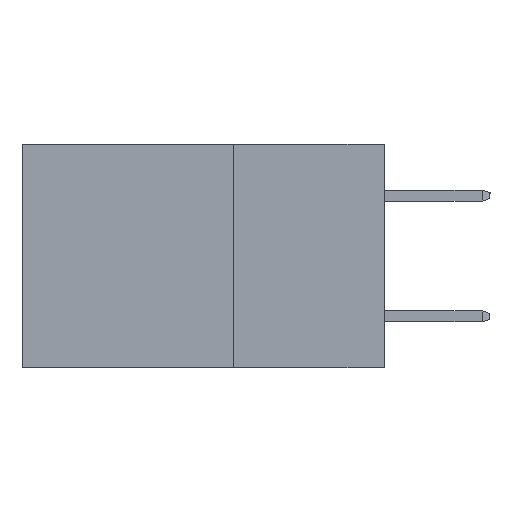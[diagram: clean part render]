
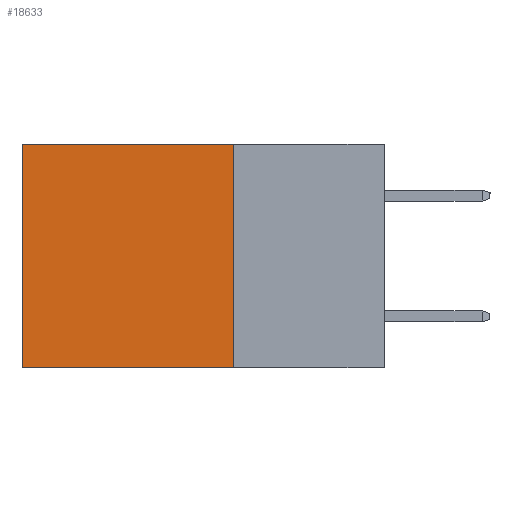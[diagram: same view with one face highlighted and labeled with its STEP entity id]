
A CAD part, left-side view. The second image highlights one B-rep face of the part: STEP entity #18633.
In plain terms, the highlighted planar face has unit normal (-1, 0, 0).
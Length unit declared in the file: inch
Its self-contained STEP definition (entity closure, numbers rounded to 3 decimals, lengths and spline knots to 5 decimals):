
#569 = EDGE_CURVE ( 'NONE', #25233, #17276, #4604, .T. ) ;
#2341 = CARTESIAN_POINT ( 'NONE',  ( 0.2615, 0.6, 0. ) ) ;
#3344 = LINE ( 'NONE', #7152, #25941 ) ;
#3527 = CARTESIAN_POINT ( 'NONE',  ( 0.2615, 0.25, -0.37 ) ) ;
#4604 = LINE ( 'NONE', #23424, #6403 ) ;
#4832 = VECTOR ( 'NONE', #15853, 39.37008 ) ;
#4960 = CARTESIAN_POINT ( 'NONE',  ( 0.2615, 0.6, -0.37 ) ) ;
#5496 = EDGE_CURVE ( 'NONE', #25233, #19333, #7345, .T. ) ;
#5846 = DIRECTION ( 'NONE',  ( 0., 0., -1. ) ) ;
#6215 = EDGE_LOOP ( 'NONE', ( #10912, #23423, #11463, #14062 ) ) ;
#6403 = VECTOR ( 'NONE', #12867, 39.37008 ) ;
#7152 = CARTESIAN_POINT ( 'NONE',  ( 0.2615, 0.25, -0.37 ) ) ;
#7345 = LINE ( 'NONE', #3527, #4832 ) ;
#7699 = DIRECTION ( 'NONE',  ( 0., 1., 0. ) ) ;
#9401 = LINE ( 'NONE', #24568, #17720 ) ;
#10912 = ORIENTED_EDGE ( 'NONE', *, *, #14545, .T. ) ;
#11463 = ORIENTED_EDGE ( 'NONE', *, *, #5496, .F. ) ;
#12867 = DIRECTION ( 'NONE',  ( 0., 1., 0. ) ) ;
#14057 = EDGE_CURVE ( 'NONE', #19333, #22505, #3344, .T. ) ;
#14062 = ORIENTED_EDGE ( 'NONE', *, *, #569, .T. ) ;
#14545 = EDGE_CURVE ( 'NONE', #17276, #22505, #9401, .T. ) ;
#15853 = DIRECTION ( 'NONE',  ( 0., 0., -1. ) ) ;
#17276 = VERTEX_POINT ( 'NONE', #2341 ) ;
#17720 = VECTOR ( 'NONE', #20624, 39.37008 ) ;
#18430 = PLANE ( 'NONE',  #20411 ) ;
#18633 = ADVANCED_FACE ( 'NONE', ( #22371 ), #18430, .F. ) ;
#19333 = VERTEX_POINT ( 'NONE', #25838 ) ;
#20304 = CARTESIAN_POINT ( 'NONE',  ( 0.2615, 0.25, 0. ) ) ;
#20411 = AXIS2_PLACEMENT_3D ( 'NONE', #26701, #24398, #5846 ) ;
#20624 = DIRECTION ( 'NONE',  ( 0., 0., -1. ) ) ;
#22371 = FACE_OUTER_BOUND ( 'NONE', #6215, .T. ) ;
#22505 = VERTEX_POINT ( 'NONE', #4960 ) ;
#23423 = ORIENTED_EDGE ( 'NONE', *, *, #14057, .F. ) ;
#23424 = CARTESIAN_POINT ( 'NONE',  ( 0.2615, 0.25, 0. ) ) ;
#24398 = DIRECTION ( 'NONE',  ( 1., 0., 0. ) ) ;
#24568 = CARTESIAN_POINT ( 'NONE',  ( 0.2615, 0.6, -0.37 ) ) ;
#25233 = VERTEX_POINT ( 'NONE', #20304 ) ;
#25838 = CARTESIAN_POINT ( 'NONE',  ( 0.2615, 0.25, -0.37 ) ) ;
#25941 = VECTOR ( 'NONE', #7699, 39.37008 ) ;
#26701 = CARTESIAN_POINT ( 'NONE',  ( 0.2615, 0.25, -0.37 ) ) ;
